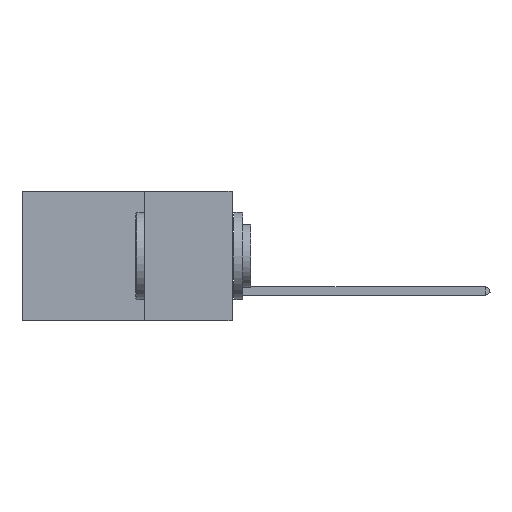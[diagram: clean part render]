
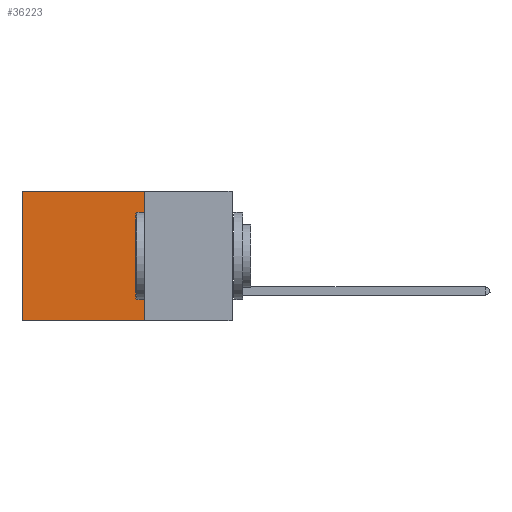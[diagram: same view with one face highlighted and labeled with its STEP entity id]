
A CAD part, left-side view. The second image highlights one B-rep face of the part: STEP entity #36223.
In plain terms, the highlighted planar face has unit normal (-1, 0, 0).
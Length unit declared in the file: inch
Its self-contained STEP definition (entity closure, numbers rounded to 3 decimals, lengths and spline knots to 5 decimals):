
#70 = ORIENTED_EDGE ( 'NONE', *, *, #1790, .T. ) ;
#555 = DIRECTION ( 'NONE',  ( 0., 1., 0. ) ) ;
#1790 = EDGE_CURVE ( 'NONE', #21978, #19075, #12404, .T. ) ;
#3347 = EDGE_CURVE ( 'NONE', #7872, #21978, #27555, .T. ) ;
#4478 = DIRECTION ( 'NONE',  ( 0., 1., 0. ) ) ;
#7819 = VECTOR ( 'NONE', #37323, 39.37008 ) ;
#7872 = VERTEX_POINT ( 'NONE', #16435 ) ;
#8386 = CARTESIAN_POINT ( 'NONE',  ( 0.2875, 0.6, 0. ) ) ;
#12404 = LINE ( 'NONE', #8386, #7819 ) ;
#13029 = VECTOR ( 'NONE', #4478, 39.37008 ) ;
#13635 = VECTOR ( 'NONE', #36756, 39.37008 ) ;
#13961 = FACE_OUTER_BOUND ( 'NONE', #15262, .T. ) ;
#14483 = PLANE ( 'NONE',  #18470 ) ;
#14863 = CARTESIAN_POINT ( 'NONE',  ( 0.2875, 0.6, 0. ) ) ;
#15262 = EDGE_LOOP ( 'NONE', ( #70, #27969, #19914, #24503 ) ) ;
#16435 = CARTESIAN_POINT ( 'NONE',  ( 0.2875, 0.25, 0. ) ) ;
#16461 = LINE ( 'NONE', #32807, #27313 ) ;
#17692 = DIRECTION ( 'NONE',  ( 0., 0., -1. ) ) ;
#18470 = AXIS2_PLACEMENT_3D ( 'NONE', #23362, #35018, #17692 ) ;
#19075 = VERTEX_POINT ( 'NONE', #25831 ) ;
#19914 = ORIENTED_EDGE ( 'NONE', *, *, #35175, .F. ) ;
#21912 = CARTESIAN_POINT ( 'NONE',  ( 0.2875, 0.25, 0. ) ) ;
#21978 = VERTEX_POINT ( 'NONE', #14863 ) ;
#23362 = CARTESIAN_POINT ( 'NONE',  ( 0.2875, 0.25, 0. ) ) ;
#24503 = ORIENTED_EDGE ( 'NONE', *, *, #3347, .T. ) ;
#25475 = CARTESIAN_POINT ( 'NONE',  ( 0.2875, 0.25, 0. ) ) ;
#25831 = CARTESIAN_POINT ( 'NONE',  ( 0.2875, 0.6, -0.37 ) ) ;
#27244 = LINE ( 'NONE', #25475, #13635 ) ;
#27313 = VECTOR ( 'NONE', #555, 39.37008 ) ;
#27555 = LINE ( 'NONE', #21912, #13029 ) ;
#27969 = ORIENTED_EDGE ( 'NONE', *, *, #29318, .F. ) ;
#29318 = EDGE_CURVE ( 'NONE', #37227, #19075, #16461, .T. ) ;
#31188 = CARTESIAN_POINT ( 'NONE',  ( 0.2875, 0.25, -0.37 ) ) ;
#32807 = CARTESIAN_POINT ( 'NONE',  ( 0.2875, 0.25, -0.37 ) ) ;
#35018 = DIRECTION ( 'NONE',  ( 1., 0., 0. ) ) ;
#35175 = EDGE_CURVE ( 'NONE', #7872, #37227, #27244, .T. ) ;
#36223 = ADVANCED_FACE ( 'NONE', ( #13961 ), #14483, .F. ) ;
#36756 = DIRECTION ( 'NONE',  ( 0., 0., -1. ) ) ;
#37227 = VERTEX_POINT ( 'NONE', #31188 ) ;
#37323 = DIRECTION ( 'NONE',  ( 0., 0., -1. ) ) ;
